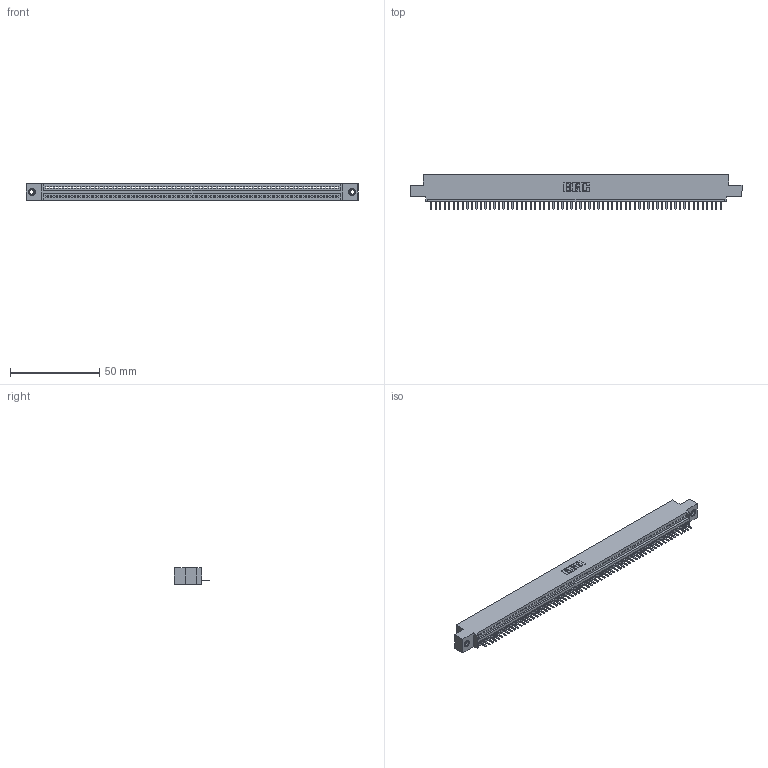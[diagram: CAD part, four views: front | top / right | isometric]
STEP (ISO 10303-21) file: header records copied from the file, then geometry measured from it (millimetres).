
FILE_DESCRIPTION (( 'STEP AP203' ), '1' );
FILE_NAME ('345-065-520-407.STEP', '2018-09-28T12:30:14', ( '' ), ( '' ), 'SwSTEP 2.0', 'SolidWorks 2016', '' );
FILE_SCHEMA (( 'CONFIG_CONTROL_DESIGN' ));
Length unit declared in the file: inch
Products named in the file (4): 345-250-001_345-250-005-103; 345-065-520-407; 345 Part_0.110 Offset - 0.156 Dia-TI; 345-292-001_345-293-120
Assembly tree (68 placements, depth 2):
  345-065-520-407
    345 Part_0.110 Offset - 0.156 Dia-TI
    345-292-001_345-293-120  x65
    345-250-001_345-250-005-103  x2
Bounding box: 186.31 x 19.68 x 9.4 mm (x, y, z)
Volume: 17610.4 mm3; surface area: 23217.9 mm2
Topology: 68 solids, 68 shells, 4220 faces, 12449 edges, 8118 vertices
Faces by surface type: plane 2846, cylinder 1358, cone 12, torus 4
Entity records: 47256 total; most frequent: CARTESIAN_POINT 8178, ORIENTED_EDGE 8158, DIRECTION 7123, EDGE_CURVE 4079, VECTOR 3663, LINE 3663, VERTEX_POINT 2712, AXIS2_PLACEMENT_3D 1730
